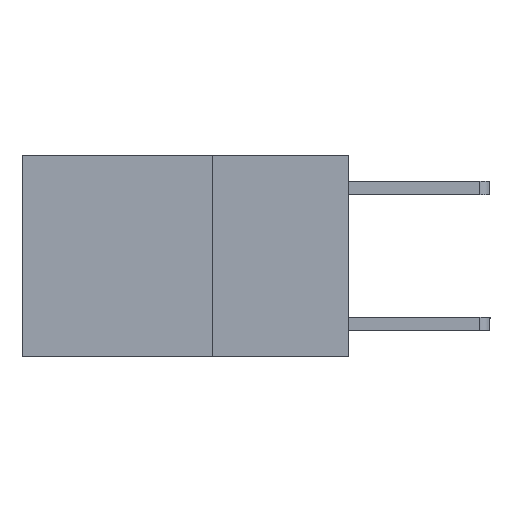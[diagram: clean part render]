
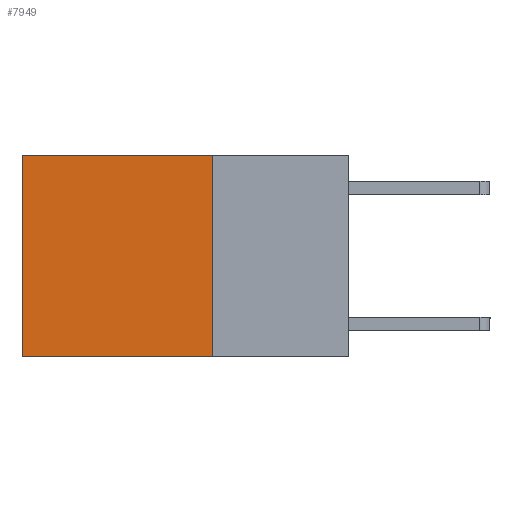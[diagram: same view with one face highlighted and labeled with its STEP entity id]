
A CAD part, left-side view. The second image highlights one B-rep face of the part: STEP entity #7949.
In plain terms, the highlighted planar face has unit normal (-1, 0, 0).
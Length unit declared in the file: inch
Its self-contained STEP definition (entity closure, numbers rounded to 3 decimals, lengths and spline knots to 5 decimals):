
#200 = EDGE_CURVE ( 'NONE', #572, #2606, #10601, .T. ) ;
#440 = EDGE_CURVE ( 'NONE', #2606, #8448, #8444, .T. ) ;
#572 = VERTEX_POINT ( 'NONE', #2854 ) ;
#747 = VERTEX_POINT ( 'NONE', #7581 ) ;
#1122 = LINE ( 'NONE', #9936, #9155 ) ;
#1155 = DIRECTION ( 'NONE',  ( 0., 1., 0. ) ) ;
#1859 = DIRECTION ( 'NONE',  ( 0., 0., -1. ) ) ;
#2168 = CARTESIAN_POINT ( 'NONE',  ( 0.2625, 0.6, 0. ) ) ;
#2606 = VERTEX_POINT ( 'NONE', #5631 ) ;
#2609 = LINE ( 'NONE', #7582, #6710 ) ;
#2734 = ORIENTED_EDGE ( 'NONE', *, *, #440, .T. ) ;
#2814 = ORIENTED_EDGE ( 'NONE', *, *, #3016, .F. ) ;
#2847 = ORIENTED_EDGE ( 'NONE', *, *, #5724, .F. ) ;
#2854 = CARTESIAN_POINT ( 'NONE',  ( 0.2625, 0.25, 0. ) ) ;
#3016 = EDGE_CURVE ( 'NONE', #747, #8448, #1122, .T. ) ;
#3386 = ORIENTED_EDGE ( 'NONE', *, *, #200, .T. ) ;
#3868 = DIRECTION ( 'NONE',  ( 1., 0., 0. ) ) ;
#4461 = DIRECTION ( 'NONE',  ( 0., 0., -1. ) ) ;
#5631 = CARTESIAN_POINT ( 'NONE',  ( 0.2625, 0.6, 0. ) ) ;
#5724 = EDGE_CURVE ( 'NONE', #572, #747, #2609, .T. ) ;
#5855 = CARTESIAN_POINT ( 'NONE',  ( 0.2625, 0.25, 0. ) ) ;
#6183 = VECTOR ( 'NONE', #4461, 39.37008 ) ;
#6412 = FACE_OUTER_BOUND ( 'NONE', #10508, .T. ) ;
#6710 = VECTOR ( 'NONE', #1859, 39.37008 ) ;
#7151 = CARTESIAN_POINT ( 'NONE',  ( 0.2625, 0.25, 0. ) ) ;
#7213 = CARTESIAN_POINT ( 'NONE',  ( 0.2625, 0.6, -0.37 ) ) ;
#7581 = CARTESIAN_POINT ( 'NONE',  ( 0.2625, 0.25, -0.37 ) ) ;
#7582 = CARTESIAN_POINT ( 'NONE',  ( 0.2625, 0.25, 0. ) ) ;
#7767 = VECTOR ( 'NONE', #7912, 39.37008 ) ;
#7912 = DIRECTION ( 'NONE',  ( 0., 1., 0. ) ) ;
#7949 = ADVANCED_FACE ( 'NONE', ( #6412 ), #8030, .F. ) ;
#8030 = PLANE ( 'NONE',  #9999 ) ;
#8444 = LINE ( 'NONE', #2168, #6183 ) ;
#8448 = VERTEX_POINT ( 'NONE', #7213 ) ;
#9155 = VECTOR ( 'NONE', #1155, 39.37008 ) ;
#9695 = DIRECTION ( 'NONE',  ( 0., 0., -1. ) ) ;
#9936 = CARTESIAN_POINT ( 'NONE',  ( 0.2625, 0.25, -0.37 ) ) ;
#9999 = AXIS2_PLACEMENT_3D ( 'NONE', #7151, #3868, #9695 ) ;
#10508 = EDGE_LOOP ( 'NONE', ( #2734, #2814, #2847, #3386 ) ) ;
#10601 = LINE ( 'NONE', #5855, #7767 ) ;
